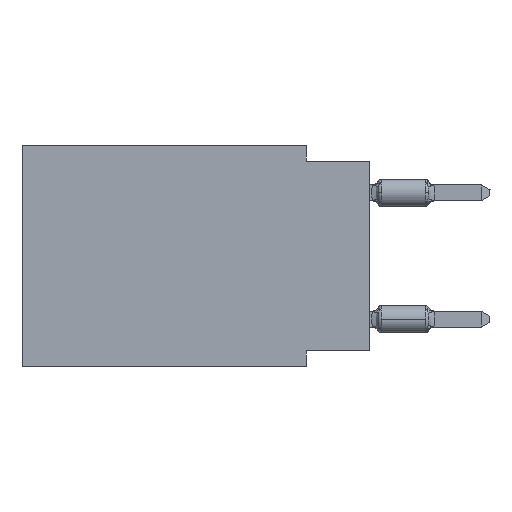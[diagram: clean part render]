
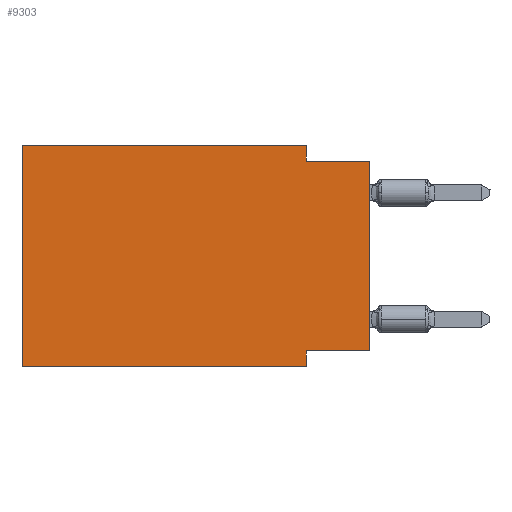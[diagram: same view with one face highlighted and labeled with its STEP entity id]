
A CAD part, left-side view. The second image highlights one B-rep face of the part: STEP entity #9303.
In plain terms, the highlighted planar face has unit normal (-1, 0, 0).
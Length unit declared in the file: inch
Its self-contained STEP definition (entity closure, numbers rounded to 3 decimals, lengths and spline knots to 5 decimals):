
#604 = LINE ( 'NONE', #21420, #2963 ) ;
#1164 = DIRECTION ( 'NONE',  ( 0., 0., 1. ) ) ;
#1395 = LINE ( 'NONE', #9860, #17002 ) ;
#1834 = LINE ( 'NONE', #22937, #24891 ) ;
#1953 = EDGE_LOOP ( 'NONE', ( #13050, #6133, #6187, #23220, #21937, #18044, #23051, #17935 ) ) ;
#2401 = DIRECTION ( 'NONE',  ( 0., -1., 0. ) ) ;
#2415 = CARTESIAN_POINT ( 'NONE',  ( 0., 0., -0.025 ) ) ;
#2963 = VECTOR ( 'NONE', #2401, 39.37008 ) ;
#3105 = LINE ( 'NONE', #11290, #10705 ) ;
#3402 = DIRECTION ( 'NONE',  ( 0., 0., -1. ) ) ;
#3906 = EDGE_CURVE ( 'NONE', #20776, #12052, #604, .T. ) ;
#4674 = VERTEX_POINT ( 'NONE', #25454 ) ;
#5558 = VERTEX_POINT ( 'NONE', #17756 ) ;
#5684 = DIRECTION ( 'NONE',  ( 0., 0., -1. ) ) ;
#6133 = ORIENTED_EDGE ( 'NONE', *, *, #11101, .F. ) ;
#6187 = ORIENTED_EDGE ( 'NONE', *, *, #19922, .F. ) ;
#6269 = VERTEX_POINT ( 'NONE', #2415 ) ;
#7619 = EDGE_CURVE ( 'NONE', #15325, #15395, #13128, .T. ) ;
#7699 = PLANE ( 'NONE',  #23944 ) ;
#8363 = CARTESIAN_POINT ( 'NONE',  ( 0., 0.1, -0.35 ) ) ;
#8849 = EDGE_CURVE ( 'NONE', #5558, #4674, #13968, .T. ) ;
#9303 = ADVANCED_FACE ( 'NONE', ( #15617 ), #7699, .F. ) ;
#9620 = DIRECTION ( 'NONE',  ( 0., -1., 0. ) ) ;
#9860 = CARTESIAN_POINT ( 'NONE',  ( 0., 0.1, 0. ) ) ;
#10705 = VECTOR ( 'NONE', #23921, 39.37008 ) ;
#11101 = EDGE_CURVE ( 'NONE', #13224, #6269, #1834, .T. ) ;
#11290 = CARTESIAN_POINT ( 'NONE',  ( 0., 0.1, -0.35 ) ) ;
#11660 = VECTOR ( 'NONE', #14807, 39.37008 ) ;
#11747 = CARTESIAN_POINT ( 'NONE',  ( 0., 0.55, 0. ) ) ;
#12010 = VECTOR ( 'NONE', #1164, 39.37008 ) ;
#12052 = VERTEX_POINT ( 'NONE', #17039 ) ;
#12742 = EDGE_CURVE ( 'NONE', #4674, #15395, #3105, .T. ) ;
#12856 = EDGE_CURVE ( 'NONE', #5558, #6269, #22115, .T. ) ;
#13050 = ORIENTED_EDGE ( 'NONE', *, *, #12856, .T. ) ;
#13128 = LINE ( 'NONE', #18075, #14525 ) ;
#13147 = CARTESIAN_POINT ( 'NONE',  ( 0., 0.55, -0.35 ) ) ;
#13224 = VERTEX_POINT ( 'NONE', #15822 ) ;
#13968 = LINE ( 'NONE', #15787, #25685 ) ;
#14525 = VECTOR ( 'NONE', #9620, 39.37008 ) ;
#14734 = LINE ( 'NONE', #23295, #11660 ) ;
#14807 = DIRECTION ( 'NONE',  ( 0., 0., 1. ) ) ;
#15088 = EDGE_CURVE ( 'NONE', #15325, #20776, #14734, .T. ) ;
#15325 = VERTEX_POINT ( 'NONE', #13147 ) ;
#15395 = VERTEX_POINT ( 'NONE', #8363 ) ;
#15617 = FACE_OUTER_BOUND ( 'NONE', #1953, .T. ) ;
#15787 = CARTESIAN_POINT ( 'NONE',  ( 0., 0., -0.325 ) ) ;
#15822 = CARTESIAN_POINT ( 'NONE',  ( 0., 0.1, -0.025 ) ) ;
#17002 = VECTOR ( 'NONE', #5684, 39.37008 ) ;
#17039 = CARTESIAN_POINT ( 'NONE',  ( 0., 0.1, 0. ) ) ;
#17756 = CARTESIAN_POINT ( 'NONE',  ( 0., 0., -0.325 ) ) ;
#17935 = ORIENTED_EDGE ( 'NONE', *, *, #8849, .F. ) ;
#18044 = ORIENTED_EDGE ( 'NONE', *, *, #7619, .T. ) ;
#18075 = CARTESIAN_POINT ( 'NONE',  ( 0., 0.55, -0.35 ) ) ;
#19922 = EDGE_CURVE ( 'NONE', #12052, #13224, #1395, .T. ) ;
#20722 = DIRECTION ( 'NONE',  ( 0., -1., 0. ) ) ;
#20776 = VERTEX_POINT ( 'NONE', #11747 ) ;
#21420 = CARTESIAN_POINT ( 'NONE',  ( 0., 0.55, 0. ) ) ;
#21937 = ORIENTED_EDGE ( 'NONE', *, *, #15088, .F. ) ;
#22115 = LINE ( 'NONE', #22248, #12010 ) ;
#22248 = CARTESIAN_POINT ( 'NONE',  ( 0., 0., 0. ) ) ;
#22421 = DIRECTION ( 'NONE',  ( 1., 0., 0. ) ) ;
#22937 = CARTESIAN_POINT ( 'NONE',  ( 0., 0., -0.025 ) ) ;
#23051 = ORIENTED_EDGE ( 'NONE', *, *, #12742, .F. ) ;
#23220 = ORIENTED_EDGE ( 'NONE', *, *, #3906, .F. ) ;
#23295 = CARTESIAN_POINT ( 'NONE',  ( 0., 0.55, 0. ) ) ;
#23921 = DIRECTION ( 'NONE',  ( 0., 0., -1. ) ) ;
#23944 = AXIS2_PLACEMENT_3D ( 'NONE', #24088, #22421, #3402 ) ;
#24088 = CARTESIAN_POINT ( 'NONE',  ( 0., 0.55, 0. ) ) ;
#24249 = DIRECTION ( 'NONE',  ( 0., 1., 0. ) ) ;
#24891 = VECTOR ( 'NONE', #20722, 39.37008 ) ;
#25454 = CARTESIAN_POINT ( 'NONE',  ( 0., 0.1, -0.325 ) ) ;
#25685 = VECTOR ( 'NONE', #24249, 39.37008 ) ;
